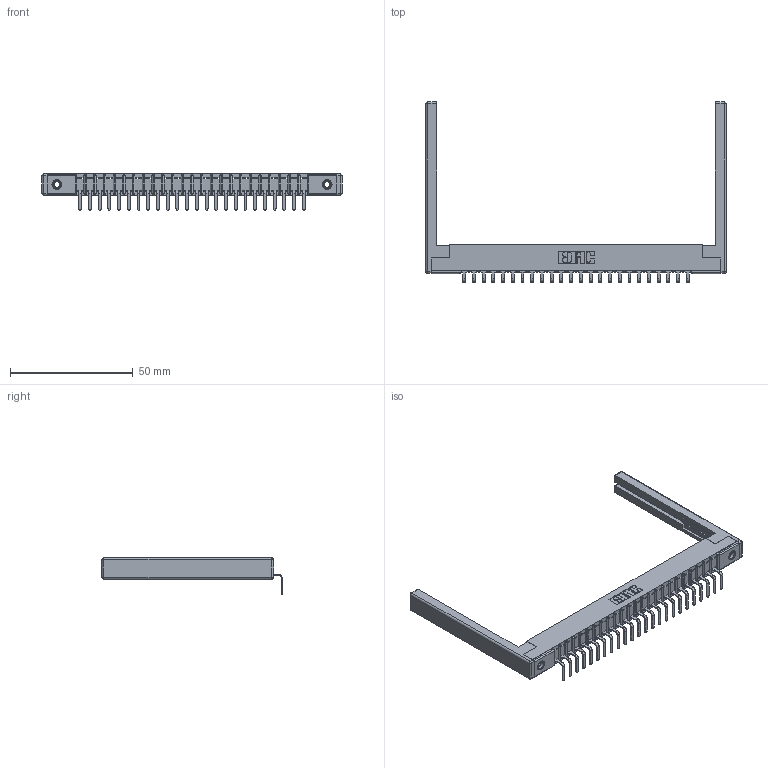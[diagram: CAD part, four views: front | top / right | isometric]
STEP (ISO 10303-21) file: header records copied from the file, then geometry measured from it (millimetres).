
FILE_DESCRIPTION (( 'STEP AP203' ), '1' );
FILE_NAME ('307-024-559-168.STEP', '2019-09-04T16:26:47', ( '' ), ( '' ), 'SwSTEP 2.0', 'SolidWorks 2016', '' );
FILE_SCHEMA (( 'CONFIG_CONTROL_DESIGN' ));
Length unit declared in the file: inch
Products named in the file (5): 307-220-068; 307 Part_.156 Dia Mounting Holes; 307-024-559-168; 307-290-001_558 559 - 1 (Single); 345-250-001_345-250-001-102
Assembly tree (29 placements, depth 2):
  307-024-559-168
    307 Part_.156 Dia Mounting Holes
    307-290-001_558 559 - 1 (Single)  x24
    307-220-068  x2
    345-250-001_345-250-001-102  x2
Bounding box: 122.53 x 73.42 x 14.81 mm (x, y, z)
Volume: 12331.9 mm3; surface area: 16398 mm2
Topology: 29 solids, 29 shells, 1737 faces, 4889 edges, 3138 vertices
Faces by surface type: plane 1094, cylinder 569, sphere 58, cone 12, torus 4
Entity records: 25657 total; most frequent: CARTESIAN_POINT 4281, ORIENTED_EDGE 4256, DIRECTION 4192, EDGE_CURVE 2128, LINE 1622, VECTOR 1622, VERTEX_POINT 1374, AXIS2_PLACEMENT_3D 1285
